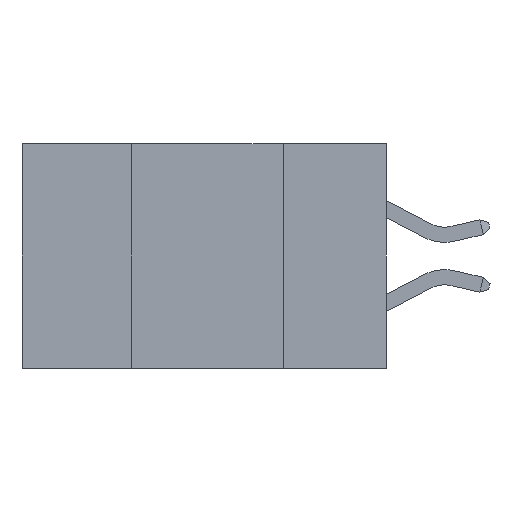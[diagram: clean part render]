
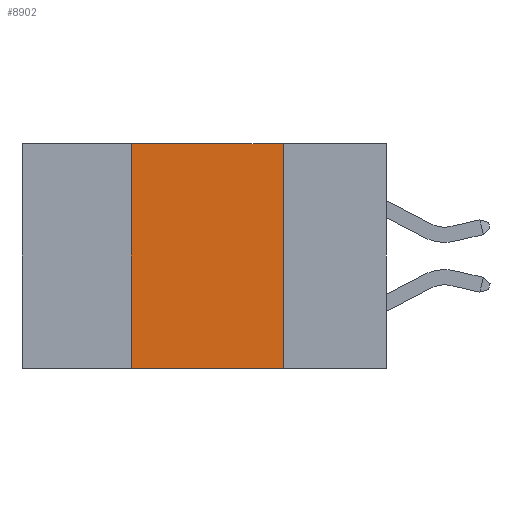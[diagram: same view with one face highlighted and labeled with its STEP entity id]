
A CAD part, left-side view. The second image highlights one B-rep face of the part: STEP entity #8902.
In plain terms, the highlighted planar face has unit normal (-1, 0, 0).
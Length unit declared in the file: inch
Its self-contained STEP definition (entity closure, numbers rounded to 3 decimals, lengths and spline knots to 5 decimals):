
#585 = VECTOR ( 'NONE', #7050, 39.37008 ) ;
#716 = LINE ( 'NONE', #4238, #585 ) ;
#738 = VECTOR ( 'NONE', #6597, 39.37008 ) ;
#878 = VECTOR ( 'NONE', #11288, 39.37008 ) ;
#973 = LINE ( 'NONE', #9164, #8935 ) ;
#1020 = PLANE ( 'NONE',  #5174 ) ;
#1341 = VERTEX_POINT ( 'NONE', #6821 ) ;
#1642 = CARTESIAN_POINT ( 'NONE',  ( 0., 0.42, 0. ) ) ;
#1933 = DIRECTION ( 'NONE',  ( 1., 0., 0. ) ) ;
#1936 = ORIENTED_EDGE ( 'NONE', *, *, #5613, .F. ) ;
#2273 = DIRECTION ( 'NONE',  ( 0., 0., 1. ) ) ;
#2822 = CARTESIAN_POINT ( 'NONE',  ( 0., 0.42, -0.37 ) ) ;
#2894 = DIRECTION ( 'NONE',  ( 0., 0., -1. ) ) ;
#4208 = ORIENTED_EDGE ( 'NONE', *, *, #4642, .F. ) ;
#4238 = CARTESIAN_POINT ( 'NONE',  ( 0., 0.6, -0.37 ) ) ;
#4330 = VERTEX_POINT ( 'NONE', #1642 ) ;
#4441 = VERTEX_POINT ( 'NONE', #2822 ) ;
#4521 = LINE ( 'NONE', #5205, #878 ) ;
#4642 = EDGE_CURVE ( 'NONE', #8247, #1341, #11195, .T. ) ;
#5174 = AXIS2_PLACEMENT_3D ( 'NONE', #9140, #1933, #2894 ) ;
#5205 = CARTESIAN_POINT ( 'NONE',  ( 0., 0.6, 0. ) ) ;
#5613 = EDGE_CURVE ( 'NONE', #4330, #8247, #4521, .T. ) ;
#6205 = ORIENTED_EDGE ( 'NONE', *, *, #6472, .T. ) ;
#6454 = ORIENTED_EDGE ( 'NONE', *, *, #7620, .F. ) ;
#6472 = EDGE_CURVE ( 'NONE', #4441, #1341, #716, .T. ) ;
#6521 = FACE_OUTER_BOUND ( 'NONE', #10128, .T. ) ;
#6597 = DIRECTION ( 'NONE',  ( 0., 0., -1. ) ) ;
#6821 = CARTESIAN_POINT ( 'NONE',  ( 0., 0.17, -0.37 ) ) ;
#7050 = DIRECTION ( 'NONE',  ( 0., -1., 0. ) ) ;
#7620 = EDGE_CURVE ( 'NONE', #4441, #4330, #973, .T. ) ;
#8247 = VERTEX_POINT ( 'NONE', #10026 ) ;
#8902 = ADVANCED_FACE ( 'NONE', ( #6521 ), #1020, .F. ) ;
#8935 = VECTOR ( 'NONE', #2273, 39.37008 ) ;
#9140 = CARTESIAN_POINT ( 'NONE',  ( 0., 0.6, 0. ) ) ;
#9164 = CARTESIAN_POINT ( 'NONE',  ( 0., 0.42, 0. ) ) ;
#10026 = CARTESIAN_POINT ( 'NONE',  ( 0., 0.17, 0. ) ) ;
#10128 = EDGE_LOOP ( 'NONE', ( #4208, #1936, #6454, #6205 ) ) ;
#10843 = CARTESIAN_POINT ( 'NONE',  ( 0., 0.17, 0. ) ) ;
#11195 = LINE ( 'NONE', #10843, #738 ) ;
#11288 = DIRECTION ( 'NONE',  ( 0., -1., 0. ) ) ;
